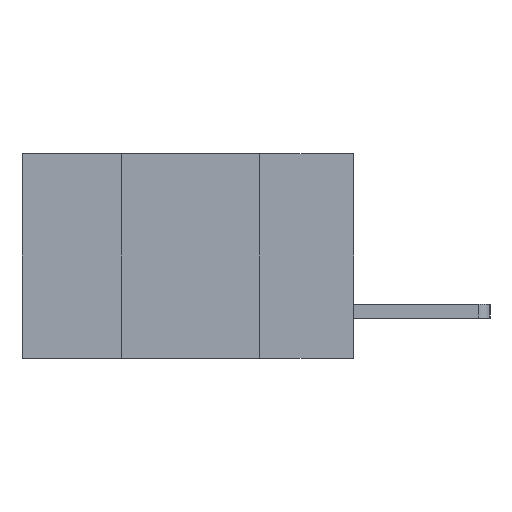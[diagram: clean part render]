
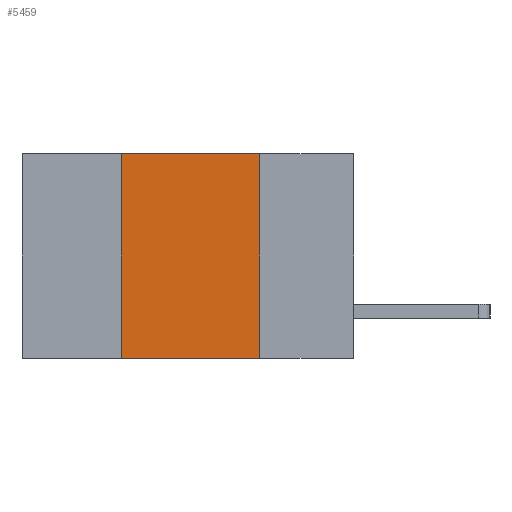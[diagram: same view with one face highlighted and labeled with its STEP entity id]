
A CAD part, left-side view. The second image highlights one B-rep face of the part: STEP entity #5459.
In plain terms, the highlighted planar face has unit normal (-1, 0, 0).
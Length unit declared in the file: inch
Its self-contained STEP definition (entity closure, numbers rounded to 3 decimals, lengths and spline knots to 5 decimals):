
#108 = LINE ( 'NONE', #1897, #8826 ) ;
#159 = PLANE ( 'NONE',  #238 ) ;
#238 = AXIS2_PLACEMENT_3D ( 'NONE', #5788, #2501, #4149 ) ;
#415 = DIRECTION ( 'NONE',  ( 0., -1., 0. ) ) ;
#845 = ORIENTED_EDGE ( 'NONE', *, *, #9196, .F. ) ;
#891 = DIRECTION ( 'NONE',  ( 0., 0., 1. ) ) ;
#1441 = EDGE_CURVE ( 'NONE', #3177, #6806, #6538, .T. ) ;
#1496 = VERTEX_POINT ( 'NONE', #8239 ) ;
#1501 = DIRECTION ( 'NONE',  ( 0., -1., 0. ) ) ;
#1897 = CARTESIAN_POINT ( 'NONE',  ( 0., 0.42, 0. ) ) ;
#2501 = DIRECTION ( 'NONE',  ( 1., 0., 0. ) ) ;
#2848 = ORIENTED_EDGE ( 'NONE', *, *, #1441, .F. ) ;
#3041 = EDGE_CURVE ( 'NONE', #6591, #3177, #8555, .T. ) ;
#3177 = VERTEX_POINT ( 'NONE', #4006 ) ;
#3746 = EDGE_CURVE ( 'NONE', #1496, #6806, #7909, .T. ) ;
#4006 = CARTESIAN_POINT ( 'NONE',  ( 0., 0.17, 0. ) ) ;
#4149 = DIRECTION ( 'NONE',  ( 0., 0., -1. ) ) ;
#4563 = VECTOR ( 'NONE', #1501, 39.37008 ) ;
#4647 = CARTESIAN_POINT ( 'NONE',  ( 0., 0.6, 0. ) ) ;
#5445 = CARTESIAN_POINT ( 'NONE',  ( 0., 0.17, -0.37 ) ) ;
#5459 = ADVANCED_FACE ( 'NONE', ( #8171 ), #159, .F. ) ;
#5760 = DIRECTION ( 'NONE',  ( 0., 0., -1. ) ) ;
#5788 = CARTESIAN_POINT ( 'NONE',  ( 0., 0.6, 0. ) ) ;
#6538 = LINE ( 'NONE', #7503, #8478 ) ;
#6591 = VERTEX_POINT ( 'NONE', #7299 ) ;
#6806 = VERTEX_POINT ( 'NONE', #5445 ) ;
#7012 = CARTESIAN_POINT ( 'NONE',  ( 0., 0.6, -0.37 ) ) ;
#7257 = VECTOR ( 'NONE', #415, 39.37008 ) ;
#7299 = CARTESIAN_POINT ( 'NONE',  ( 0., 0.42, 0. ) ) ;
#7503 = CARTESIAN_POINT ( 'NONE',  ( 0., 0.17, 0. ) ) ;
#7909 = LINE ( 'NONE', #7012, #4563 ) ;
#8050 = ORIENTED_EDGE ( 'NONE', *, *, #3746, .T. ) ;
#8171 = FACE_OUTER_BOUND ( 'NONE', #8776, .T. ) ;
#8239 = CARTESIAN_POINT ( 'NONE',  ( 0., 0.42, -0.37 ) ) ;
#8478 = VECTOR ( 'NONE', #5760, 39.37008 ) ;
#8496 = ORIENTED_EDGE ( 'NONE', *, *, #3041, .F. ) ;
#8555 = LINE ( 'NONE', #4647, #7257 ) ;
#8776 = EDGE_LOOP ( 'NONE', ( #2848, #8496, #845, #8050 ) ) ;
#8826 = VECTOR ( 'NONE', #891, 39.37008 ) ;
#9196 = EDGE_CURVE ( 'NONE', #1496, #6591, #108, .T. ) ;
